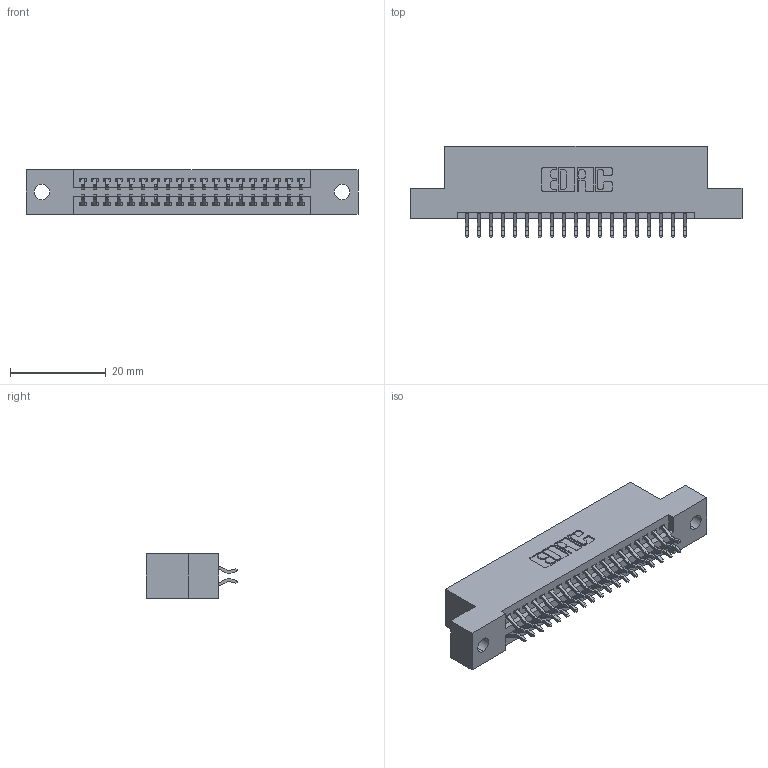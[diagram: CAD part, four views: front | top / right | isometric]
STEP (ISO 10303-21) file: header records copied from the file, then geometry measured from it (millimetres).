
FILE_DESCRIPTION (( 'STEP AP203' ), '1' );
FILE_NAME ('345-038-556-202.STEP', '2019-10-28T15:47:45', ( '' ), ( '' ), 'SwSTEP 2.0', 'SolidWorks 2016', '' );
FILE_SCHEMA (( 'CONFIG_CONTROL_DESIGN' ));
Length unit declared in the file: inch
Products named in the file (3): 345 Part_Flush Mounting Lugs - 0.128 Dia; 345-292-001_556 Tail; 345-038-556-202
Assembly tree (39 placements, depth 2):
  345-038-556-202
    345 Part_Flush Mounting Lugs - 0.128 Dia
    345-292-001_556 Tail  x38
Bounding box: 69.47 x 19.24 x 9.4 mm (x, y, z)
Volume: 6496.6 mm3; surface area: 8851.6 mm2
Topology: 39 solids, 39 shells, 2254 faces, 6687 edges, 4406 vertices
Faces by surface type: plane 1486, cylinder 768
Entity records: 18227 total; most frequent: CARTESIAN_POINT 3092, ORIENTED_EDGE 3014, DIRECTION 2743, EDGE_CURVE 1507, LINE 1291, VECTOR 1291, VERTEX_POINT 1002, AXIS2_PLACEMENT_3D 726
